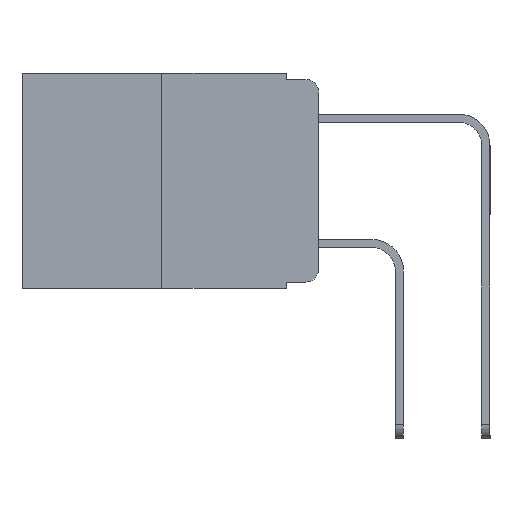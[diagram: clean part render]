
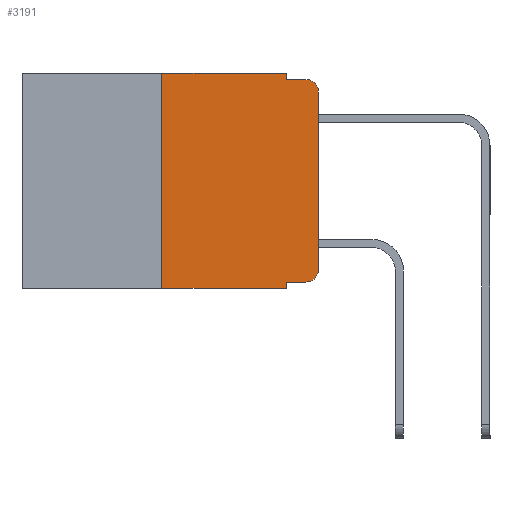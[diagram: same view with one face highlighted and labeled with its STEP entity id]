
A CAD part, left-side view. The second image highlights one B-rep face of the part: STEP entity #3191.
In plain terms, the highlighted planar face has unit normal (-1, 0, 0).
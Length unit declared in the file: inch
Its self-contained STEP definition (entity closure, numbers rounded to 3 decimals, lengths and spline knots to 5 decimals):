
#65 = CARTESIAN_POINT ( 'NONE',  ( 0., 0.051, -0.343 ) ) ;
#270 = EDGE_CURVE ( 'NONE', #1262, #4531, #14368, .T. ) ;
#288 = CARTESIAN_POINT ( 'NONE',  ( 0., 0.473, -0.343 ) ) ;
#370 = CARTESIAN_POINT ( 'NONE',  ( 0., 0.25, 0. ) ) ;
#993 = LINE ( 'NONE', #14868, #16413 ) ;
#1056 = FACE_OUTER_BOUND ( 'NONE', #6675, .T. ) ;
#1080 = VERTEX_POINT ( 'NONE', #17702 ) ;
#1262 = VERTEX_POINT ( 'NONE', #2700 ) ;
#1267 = DIRECTION ( 'NONE',  ( -1., 0., 0. ) ) ;
#1478 = CARTESIAN_POINT ( 'NONE',  ( 0., 0.02, -0.333 ) ) ;
#1571 = EDGE_CURVE ( 'NONE', #1691, #4531, #17302, .T. ) ;
#1691 = VERTEX_POINT ( 'NONE', #2798 ) ;
#2118 = VERTEX_POINT ( 'NONE', #1478 ) ;
#2154 = CARTESIAN_POINT ( 'NONE',  ( 0., 0., 0. ) ) ;
#2203 = CARTESIAN_POINT ( 'NONE',  ( 0., 0.473, 0. ) ) ;
#2488 = DIRECTION ( 'NONE',  ( 0., -1., 0. ) ) ;
#2692 = EDGE_CURVE ( 'NONE', #1262, #3256, #12772, .T. ) ;
#2700 = CARTESIAN_POINT ( 'NONE',  ( 0., 0.25, -0.343 ) ) ;
#2798 = CARTESIAN_POINT ( 'NONE',  ( 0., 0.051, -0.333 ) ) ;
#3191 = ADVANCED_FACE ( 'NONE', ( #1056 ), #8286, .F. ) ;
#3256 = VERTEX_POINT ( 'NONE', #370 ) ;
#3305 = LINE ( 'NONE', #2203, #12151 ) ;
#3632 = VERTEX_POINT ( 'NONE', #17311 ) ;
#3882 = DIRECTION ( 'NONE',  ( 0., 0., -1. ) ) ;
#3960 = VECTOR ( 'NONE', #6024, 39.37008 ) ;
#3978 = CARTESIAN_POINT ( 'NONE',  ( 0., 0.051, 0. ) ) ;
#4194 = VERTEX_POINT ( 'NONE', #7613 ) ;
#4531 = VERTEX_POINT ( 'NONE', #65 ) ;
#4837 = ORIENTED_EDGE ( 'NONE', *, *, #16267, .T. ) ;
#6024 = DIRECTION ( 'NONE',  ( 0., 0., 1. ) ) ;
#6067 = EDGE_CURVE ( 'NONE', #20976, #13906, #10920, .T. ) ;
#6146 = ORIENTED_EDGE ( 'NONE', *, *, #11620, .T. ) ;
#6192 = VECTOR ( 'NONE', #6834, 39.37008 ) ;
#6500 = VECTOR ( 'NONE', #20056, 39.37008 ) ;
#6675 = EDGE_LOOP ( 'NONE', ( #10055, #6146, #19050, #6677, #15332, #15821, #20047, #8298, #13096, #4837 ) ) ;
#6677 = ORIENTED_EDGE ( 'NONE', *, *, #6067, .F. ) ;
#6706 = CARTESIAN_POINT ( 'NONE',  ( 0., 0.25, 0. ) ) ;
#6834 = DIRECTION ( 'NONE',  ( 0., -1., 0. ) ) ;
#7237 = EDGE_CURVE ( 'NONE', #13906, #3632, #993, .T. ) ;
#7253 = DIRECTION ( 'NONE',  ( 0., 0., 1. ) ) ;
#7426 = CARTESIAN_POINT ( 'NONE',  ( 0., 0.02, -0.03 ) ) ;
#7613 = CARTESIAN_POINT ( 'NONE',  ( 0., 0., -0.313 ) ) ;
#7972 = CIRCLE ( 'NONE', #12762, 0.02 ) ;
#8111 = EDGE_CURVE ( 'NONE', #3256, #20976, #3305, .T. ) ;
#8273 = VECTOR ( 'NONE', #3882, 39.37008 ) ;
#8286 = PLANE ( 'NONE',  #17469 ) ;
#8298 = ORIENTED_EDGE ( 'NONE', *, *, #1571, .F. ) ;
#8501 = AXIS2_PLACEMENT_3D ( 'NONE', #11261, #1267, #12873 ) ;
#8559 = DIRECTION ( 'NONE',  ( 0., 0., -1. ) ) ;
#8675 = DIRECTION ( 'NONE',  ( 1., 0., 0. ) ) ;
#8871 = VECTOR ( 'NONE', #11752, 39.37008 ) ;
#9105 = DIRECTION ( 'NONE',  ( 0., 0., -1. ) ) ;
#9213 = CARTESIAN_POINT ( 'NONE',  ( 0., 0.473, 0. ) ) ;
#9491 = DIRECTION ( 'NONE',  ( 0., -1., 0. ) ) ;
#10055 = ORIENTED_EDGE ( 'NONE', *, *, #12696, .T. ) ;
#10920 = LINE ( 'NONE', #20042, #6500 ) ;
#11261 = CARTESIAN_POINT ( 'NONE',  ( 0., 0.02, -0.313 ) ) ;
#11620 = EDGE_CURVE ( 'NONE', #1080, #3632, #7972, .T. ) ;
#11689 = CARTESIAN_POINT ( 'NONE',  ( 0., 0.051, -0.333 ) ) ;
#11752 = DIRECTION ( 'NONE',  ( 0., -1., 0. ) ) ;
#12151 = VECTOR ( 'NONE', #2488, 39.37008 ) ;
#12696 = EDGE_CURVE ( 'NONE', #4194, #1080, #19939, .T. ) ;
#12762 = AXIS2_PLACEMENT_3D ( 'NONE', #7426, #18677, #9105 ) ;
#12772 = LINE ( 'NONE', #6706, #3960 ) ;
#12873 = DIRECTION ( 'NONE',  ( 0., 0., -1. ) ) ;
#13096 = ORIENTED_EDGE ( 'NONE', *, *, #19469, .T. ) ;
#13141 = LINE ( 'NONE', #11689, #8871 ) ;
#13906 = VERTEX_POINT ( 'NONE', #15036 ) ;
#14080 = CIRCLE ( 'NONE', #8501, 0.02 ) ;
#14368 = LINE ( 'NONE', #288, #6192 ) ;
#14868 = CARTESIAN_POINT ( 'NONE',  ( 0., 0.051, -0.01 ) ) ;
#15036 = CARTESIAN_POINT ( 'NONE',  ( 0., 0.051, -0.01 ) ) ;
#15332 = ORIENTED_EDGE ( 'NONE', *, *, #8111, .F. ) ;
#15714 = VECTOR ( 'NONE', #7253, 39.37008 ) ;
#15821 = ORIENTED_EDGE ( 'NONE', *, *, #2692, .F. ) ;
#16267 = EDGE_CURVE ( 'NONE', #2118, #4194, #14080, .T. ) ;
#16413 = VECTOR ( 'NONE', #9491, 39.37008 ) ;
#17302 = LINE ( 'NONE', #19023, #8273 ) ;
#17311 = CARTESIAN_POINT ( 'NONE',  ( 0., 0.02, -0.01 ) ) ;
#17469 = AXIS2_PLACEMENT_3D ( 'NONE', #9213, #8675, #8559 ) ;
#17702 = CARTESIAN_POINT ( 'NONE',  ( 0., 0., -0.03 ) ) ;
#18677 = DIRECTION ( 'NONE',  ( -1., 0., 0. ) ) ;
#19023 = CARTESIAN_POINT ( 'NONE',  ( 0., 0.051, 0. ) ) ;
#19050 = ORIENTED_EDGE ( 'NONE', *, *, #7237, .F. ) ;
#19469 = EDGE_CURVE ( 'NONE', #1691, #2118, #13141, .T. ) ;
#19939 = LINE ( 'NONE', #2154, #15714 ) ;
#20042 = CARTESIAN_POINT ( 'NONE',  ( 0., 0.051, 0. ) ) ;
#20047 = ORIENTED_EDGE ( 'NONE', *, *, #270, .T. ) ;
#20056 = DIRECTION ( 'NONE',  ( 0., 0., -1. ) ) ;
#20976 = VERTEX_POINT ( 'NONE', #3978 ) ;
